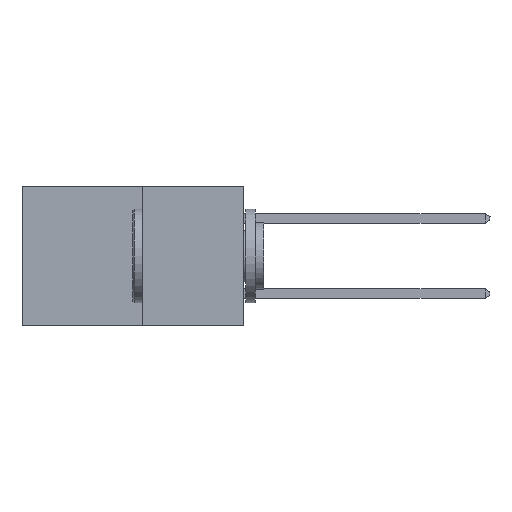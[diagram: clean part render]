
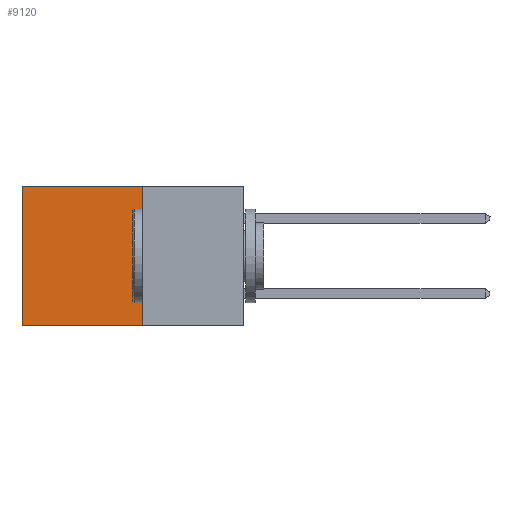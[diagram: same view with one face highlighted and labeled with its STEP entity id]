
A CAD part, left-side view. The second image highlights one B-rep face of the part: STEP entity #9120.
In plain terms, the highlighted planar face has unit normal (-1, 0, 0).
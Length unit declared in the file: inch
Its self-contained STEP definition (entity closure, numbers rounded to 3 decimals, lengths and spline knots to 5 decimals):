
#109 = CARTESIAN_POINT ( 'NONE',  ( 0.277, 0.59, -0.37 ) ) ;
#218 = ORIENTED_EDGE ( 'NONE', *, *, #353, .T. ) ;
#278 = EDGE_CURVE ( 'NONE', #9692, #14951, #15277, .T. ) ;
#353 = EDGE_CURVE ( 'NONE', #14951, #15414, #10956, .T. ) ;
#667 = EDGE_CURVE ( 'NONE', #9692, #2717, #9452, .T. ) ;
#1491 = ORIENTED_EDGE ( 'NONE', *, *, #8280, .F. ) ;
#2118 = DIRECTION ( 'NONE',  ( 0., 1., 0. ) ) ;
#2717 = VERTEX_POINT ( 'NONE', #15644 ) ;
#2982 = VECTOR ( 'NONE', #14596, 39.37008 ) ;
#4103 = AXIS2_PLACEMENT_3D ( 'NONE', #10138, #10006, #9795 ) ;
#5845 = VECTOR ( 'NONE', #10514, 39.37008 ) ;
#6901 = EDGE_LOOP ( 'NONE', ( #218, #1491, #12238, #13066 ) ) ;
#7333 = VECTOR ( 'NONE', #12668, 39.37008 ) ;
#7738 = CARTESIAN_POINT ( 'NONE',  ( 0.277, 0.59, -0.37 ) ) ;
#8280 = EDGE_CURVE ( 'NONE', #2717, #15414, #10184, .T. ) ;
#8347 = CARTESIAN_POINT ( 'NONE',  ( 0.277, 0.27, -0.37 ) ) ;
#9120 = ADVANCED_FACE ( 'NONE', ( #11670 ), #10203, .F. ) ;
#9452 = LINE ( 'NONE', #17219, #5845 ) ;
#9692 = VERTEX_POINT ( 'NONE', #10849 ) ;
#9795 = DIRECTION ( 'NONE',  ( 0., 0., -1. ) ) ;
#10006 = DIRECTION ( 'NONE',  ( 1., 0., 0. ) ) ;
#10138 = CARTESIAN_POINT ( 'NONE',  ( 0.277, 0.27, -0.37 ) ) ;
#10184 = LINE ( 'NONE', #8347, #2982 ) ;
#10203 = PLANE ( 'NONE',  #4103 ) ;
#10514 = DIRECTION ( 'NONE',  ( 0., 0., -1. ) ) ;
#10849 = CARTESIAN_POINT ( 'NONE',  ( 0.277, 0.27, 0. ) ) ;
#10956 = LINE ( 'NONE', #109, #7333 ) ;
#11361 = CARTESIAN_POINT ( 'NONE',  ( 0.277, 0.59, 0. ) ) ;
#11670 = FACE_OUTER_BOUND ( 'NONE', #6901, .T. ) ;
#11774 = VECTOR ( 'NONE', #2118, 39.37008 ) ;
#12238 = ORIENTED_EDGE ( 'NONE', *, *, #667, .F. ) ;
#12668 = DIRECTION ( 'NONE',  ( 0., 0., -1. ) ) ;
#13066 = ORIENTED_EDGE ( 'NONE', *, *, #278, .T. ) ;
#14596 = DIRECTION ( 'NONE',  ( 0., 1., 0. ) ) ;
#14951 = VERTEX_POINT ( 'NONE', #11361 ) ;
#15277 = LINE ( 'NONE', #15995, #11774 ) ;
#15414 = VERTEX_POINT ( 'NONE', #7738 ) ;
#15644 = CARTESIAN_POINT ( 'NONE',  ( 0.277, 0.27, -0.37 ) ) ;
#15995 = CARTESIAN_POINT ( 'NONE',  ( 0.277, 0.27, 0. ) ) ;
#17219 = CARTESIAN_POINT ( 'NONE',  ( 0.277, 0.27, -0.37 ) ) ;
